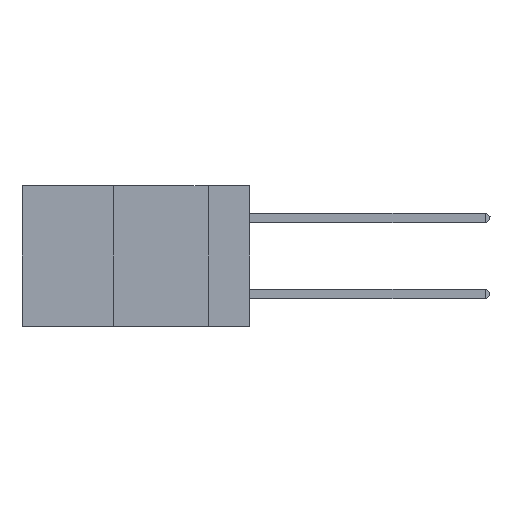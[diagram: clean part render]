
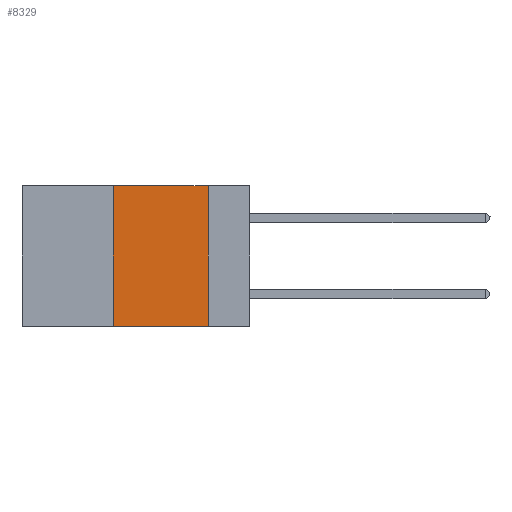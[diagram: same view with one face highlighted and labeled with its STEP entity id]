
A CAD part, left-side view. The second image highlights one B-rep face of the part: STEP entity #8329.
In plain terms, the highlighted planar face has unit normal (-1, 0, 0).
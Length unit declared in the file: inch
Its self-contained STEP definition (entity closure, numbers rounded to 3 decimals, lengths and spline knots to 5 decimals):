
#862 = CARTESIAN_POINT ( 'NONE',  ( 0., 0.11, -0.37 ) ) ;
#1023 = DIRECTION ( 'NONE',  ( 0., 0., -1. ) ) ;
#1349 = LINE ( 'NONE', #19511, #22726 ) ;
#3083 = AXIS2_PLACEMENT_3D ( 'NONE', #10625, #16214, #1023 ) ;
#8329 = ADVANCED_FACE ( 'NONE', ( #31154 ), #25792, .F. ) ;
#10193 = VECTOR ( 'NONE', #11572, 39.37008 ) ;
#10625 = CARTESIAN_POINT ( 'NONE',  ( 0., 0.6, 0. ) ) ;
#11572 = DIRECTION ( 'NONE',  ( 0., 0., -1. ) ) ;
#11573 = CARTESIAN_POINT ( 'NONE',  ( 0., 0.6, 0. ) ) ;
#11766 = LINE ( 'NONE', #11573, #23402 ) ;
#11800 = ORIENTED_EDGE ( 'NONE', *, *, #32813, .F. ) ;
#11828 = VERTEX_POINT ( 'NONE', #17907 ) ;
#11986 = DIRECTION ( 'NONE',  ( 0., 0., 1. ) ) ;
#14973 = CARTESIAN_POINT ( 'NONE',  ( 0., 0.36, 0. ) ) ;
#16214 = DIRECTION ( 'NONE',  ( 1., 0., 0. ) ) ;
#16516 = EDGE_CURVE ( 'NONE', #34477, #11828, #39298, .T. ) ;
#17159 = CARTESIAN_POINT ( 'NONE',  ( 0., 0.11, 0. ) ) ;
#17246 = ORIENTED_EDGE ( 'NONE', *, *, #28993, .T. ) ;
#17344 = VECTOR ( 'NONE', #11986, 39.37008 ) ;
#17907 = CARTESIAN_POINT ( 'NONE',  ( 0., 0.36, 0. ) ) ;
#18134 = ORIENTED_EDGE ( 'NONE', *, *, #23656, .F. ) ;
#19283 = VERTEX_POINT ( 'NONE', #862 ) ;
#19511 = CARTESIAN_POINT ( 'NONE',  ( 0., 0.6, -0.37 ) ) ;
#22726 = VECTOR ( 'NONE', #31465, 39.37008 ) ;
#23263 = CARTESIAN_POINT ( 'NONE',  ( 0., 0.36, -0.37 ) ) ;
#23402 = VECTOR ( 'NONE', #36076, 39.37008 ) ;
#23656 = EDGE_CURVE ( 'NONE', #11828, #24577, #11766, .T. ) ;
#24577 = VERTEX_POINT ( 'NONE', #34710 ) ;
#25203 = EDGE_LOOP ( 'NONE', ( #11800, #18134, #35370, #17246 ) ) ;
#25792 = PLANE ( 'NONE',  #3083 ) ;
#28993 = EDGE_CURVE ( 'NONE', #34477, #19283, #1349, .T. ) ;
#31154 = FACE_OUTER_BOUND ( 'NONE', #25203, .T. ) ;
#31465 = DIRECTION ( 'NONE',  ( 0., -1., 0. ) ) ;
#32813 = EDGE_CURVE ( 'NONE', #24577, #19283, #38871, .T. ) ;
#34477 = VERTEX_POINT ( 'NONE', #23263 ) ;
#34710 = CARTESIAN_POINT ( 'NONE',  ( 0., 0.11, 0. ) ) ;
#35370 = ORIENTED_EDGE ( 'NONE', *, *, #16516, .F. ) ;
#36076 = DIRECTION ( 'NONE',  ( 0., -1., 0. ) ) ;
#38871 = LINE ( 'NONE', #17159, #10193 ) ;
#39298 = LINE ( 'NONE', #14973, #17344 ) ;
